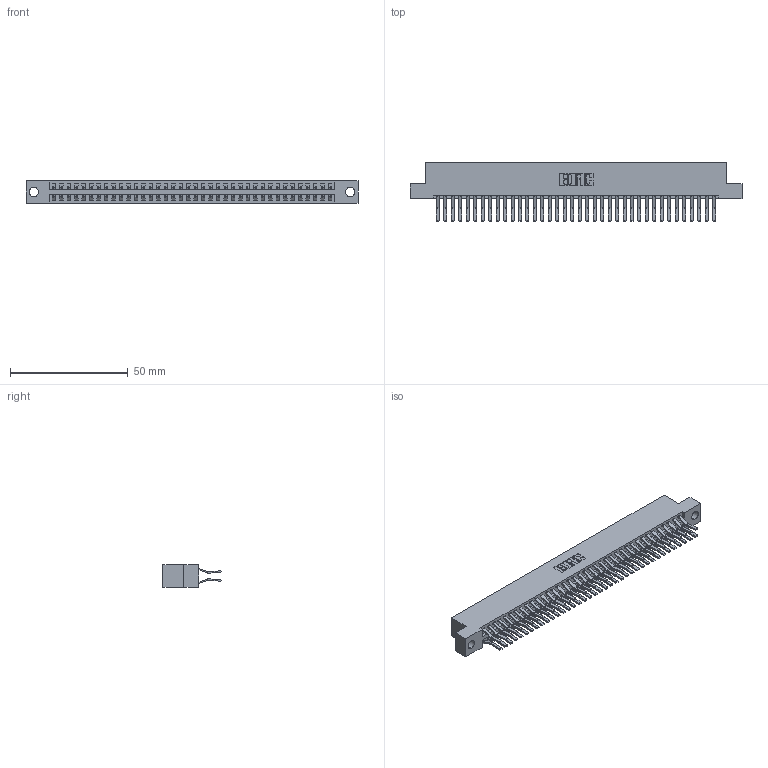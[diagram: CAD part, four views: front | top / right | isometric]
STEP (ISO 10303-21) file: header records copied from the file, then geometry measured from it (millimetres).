
FILE_DESCRIPTION (( 'STEP AP203' ), '1' );
FILE_NAME ('346-076-560-204.STEP', '2018-08-29T04:56:26', ( '' ), ( '' ), 'SwSTEP 2.0', 'SolidWorks 2016', '' );
FILE_SCHEMA (( 'CONFIG_CONTROL_DESIGN' ));
Length unit declared in the file: inch
Products named in the file (3): 346-076-560-204; 346 Part_Flush Mounting Lugs - 0.156 Dia-TH; 345-292-001_560 Tail
Assembly tree (77 placements, depth 2):
  346-076-560-204
    346 Part_Flush Mounting Lugs - 0.156 Dia-TH
    345-292-001_560 Tail  x76
Bounding box: 141.22 x 24.78 x 9.4 mm (x, y, z)
Volume: 14150.3 mm3; surface area: 20530.1 mm2
Topology: 77 solids, 77 shells, 4226 faces, 12565 edges, 8274 vertices
Faces by surface type: plane 2736, cylinder 1490
Entity records: 25429 total; most frequent: CARTESIAN_POINT 4196, ORIENTED_EDGE 4130, DIRECTION 3753, EDGE_CURVE 2065, LINE 1777, VECTOR 1777, VERTEX_POINT 1374, AXIS2_PLACEMENT_3D 988
